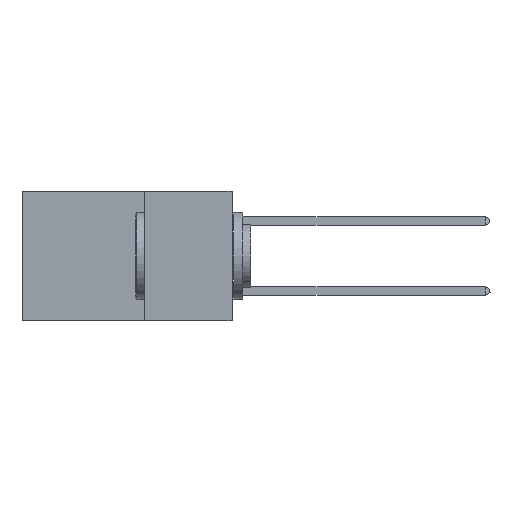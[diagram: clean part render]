
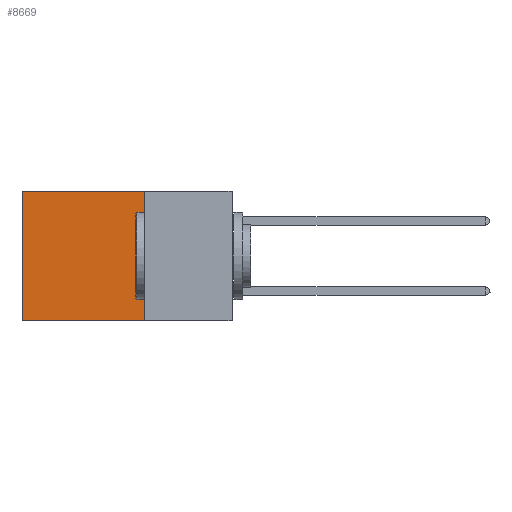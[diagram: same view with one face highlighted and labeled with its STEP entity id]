
A CAD part, left-side view. The second image highlights one B-rep face of the part: STEP entity #8669.
In plain terms, the highlighted planar face has unit normal (-1, 0, 0).
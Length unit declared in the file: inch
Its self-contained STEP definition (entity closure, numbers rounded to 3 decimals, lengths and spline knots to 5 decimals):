
#450 = PLANE ( 'NONE',  #3458 ) ;
#478 = CARTESIAN_POINT ( 'NONE',  ( 0.2875, 0.6, 0. ) ) ;
#517 = EDGE_CURVE ( 'NONE', #5654, #647, #790, .T. ) ;
#647 = VERTEX_POINT ( 'NONE', #9992 ) ;
#716 = EDGE_CURVE ( 'NONE', #647, #10250, #10219, .T. ) ;
#790 = LINE ( 'NONE', #1112, #8520 ) ;
#1112 = CARTESIAN_POINT ( 'NONE',  ( 0.2875, 0.25, 0. ) ) ;
#2230 = FACE_OUTER_BOUND ( 'NONE', #7369, .T. ) ;
#3306 = ORIENTED_EDGE ( 'NONE', *, *, #716, .T. ) ;
#3458 = AXIS2_PLACEMENT_3D ( 'NONE', #8931, #7629, #12964 ) ;
#3524 = VECTOR ( 'NONE', #4578, 39.37008 ) ;
#4578 = DIRECTION ( 'NONE',  ( 0., 0., -1. ) ) ;
#4941 = DIRECTION ( 'NONE',  ( 0., 1., 0. ) ) ;
#5654 = VERTEX_POINT ( 'NONE', #12368 ) ;
#6888 = ORIENTED_EDGE ( 'NONE', *, *, #517, .T. ) ;
#6987 = EDGE_CURVE ( 'NONE', #5654, #7973, #10061, .T. ) ;
#7369 = EDGE_LOOP ( 'NONE', ( #3306, #12173, #10309, #6888 ) ) ;
#7629 = DIRECTION ( 'NONE',  ( 1., 0., 0. ) ) ;
#7973 = VERTEX_POINT ( 'NONE', #16711 ) ;
#8361 = VECTOR ( 'NONE', #16174, 39.37008 ) ;
#8520 = VECTOR ( 'NONE', #13004, 39.37008 ) ;
#8669 = ADVANCED_FACE ( 'NONE', ( #2230 ), #450, .F. ) ;
#8931 = CARTESIAN_POINT ( 'NONE',  ( 0.2875, 0.25, 0. ) ) ;
#9992 = CARTESIAN_POINT ( 'NONE',  ( 0.2875, 0.6, 0. ) ) ;
#10061 = LINE ( 'NONE', #16234, #8361 ) ;
#10219 = LINE ( 'NONE', #478, #3524 ) ;
#10250 = VERTEX_POINT ( 'NONE', #10559 ) ;
#10309 = ORIENTED_EDGE ( 'NONE', *, *, #6987, .F. ) ;
#10559 = CARTESIAN_POINT ( 'NONE',  ( 0.2875, 0.6, -0.37 ) ) ;
#11537 = CARTESIAN_POINT ( 'NONE',  ( 0.2875, 0.25, -0.37 ) ) ;
#12173 = ORIENTED_EDGE ( 'NONE', *, *, #14114, .F. ) ;
#12368 = CARTESIAN_POINT ( 'NONE',  ( 0.2875, 0.25, 0. ) ) ;
#12964 = DIRECTION ( 'NONE',  ( 0., 0., -1. ) ) ;
#13004 = DIRECTION ( 'NONE',  ( 0., 1., 0. ) ) ;
#13547 = VECTOR ( 'NONE', #4941, 39.37008 ) ;
#14114 = EDGE_CURVE ( 'NONE', #7973, #10250, #16532, .T. ) ;
#16174 = DIRECTION ( 'NONE',  ( 0., 0., -1. ) ) ;
#16234 = CARTESIAN_POINT ( 'NONE',  ( 0.2875, 0.25, 0. ) ) ;
#16532 = LINE ( 'NONE', #11537, #13547 ) ;
#16711 = CARTESIAN_POINT ( 'NONE',  ( 0.2875, 0.25, -0.37 ) ) ;
